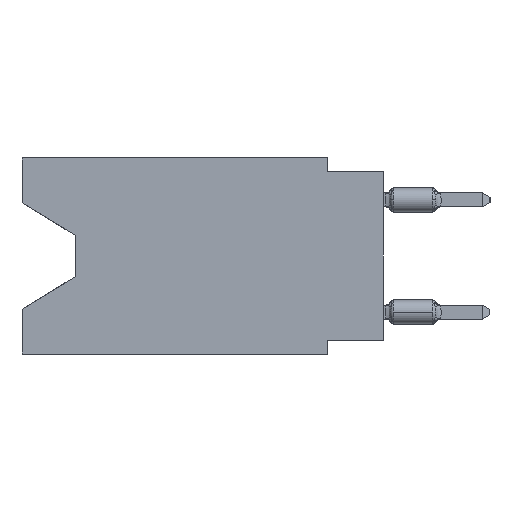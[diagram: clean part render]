
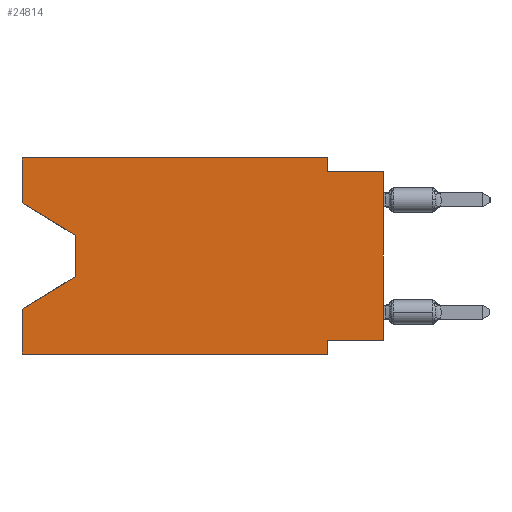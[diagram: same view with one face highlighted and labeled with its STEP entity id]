
A CAD part, left-side view. The second image highlights one B-rep face of the part: STEP entity #24814.
In plain terms, the highlighted planar face has unit normal (-1, 0, 0).
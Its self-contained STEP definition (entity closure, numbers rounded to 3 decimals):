
#382 = ORIENTED_EDGE ( 'NONE', *, *, #13523, .F. ) ;
#453 = ORIENTED_EDGE ( 'NONE', *, *, #15344, .F. ) ;
#481 = VECTOR ( 'NONE', #26315, 1000. ) ;
#1238 = LINE ( 'NONE', #21704, #481 ) ;
#2093 = VECTOR ( 'NONE', #11707, 1000. ) ;
#2851 = ORIENTED_EDGE ( 'NONE', *, *, #11258, .F. ) ;
#3063 = DIRECTION ( 'NONE',  ( 0., 0., -1. ) ) ;
#3077 = EDGE_CURVE ( 'NONE', #9585, #11407, #1238, .T. ) ;
#3196 = ORIENTED_EDGE ( 'NONE', *, *, #18572, .T. ) ;
#3495 = CARTESIAN_POINT ( 'NONE',  ( 0., 2.54, -8.255 ) ) ;
#4495 = DIRECTION ( 'NONE',  ( 0., 0., -1. ) ) ;
#4534 = DIRECTION ( 'NONE',  ( 0., 1., 0. ) ) ;
#4892 = LINE ( 'NONE', #27179, #11054 ) ;
#5324 = DIRECTION ( 'NONE',  ( 0., -1., 0. ) ) ;
#5427 = CARTESIAN_POINT ( 'NONE',  ( 0., 16.383, 0. ) ) ;
#6750 = ORIENTED_EDGE ( 'NONE', *, *, #13107, .F. ) ;
#6770 = CARTESIAN_POINT ( 'NONE',  ( 0., 16.383, 0. ) ) ;
#6858 = FACE_OUTER_BOUND ( 'NONE', #20881, .T. ) ;
#7109 = CARTESIAN_POINT ( 'NONE',  ( 0., 2.54, 0. ) ) ;
#7280 = ORIENTED_EDGE ( 'NONE', *, *, #23712, .F. ) ;
#7559 = CARTESIAN_POINT ( 'NONE',  ( 0., 0., -0.635 ) ) ;
#7583 = VERTEX_POINT ( 'NONE', #18325 ) ;
#8108 = VERTEX_POINT ( 'NONE', #23703 ) ;
#8477 = LINE ( 'NONE', #10928, #9392 ) ;
#8680 = CARTESIAN_POINT ( 'NONE',  ( 0., 16.383, -2.038 ) ) ;
#8782 = DIRECTION ( 'NONE',  ( 0., 0., -1. ) ) ;
#8787 = CARTESIAN_POINT ( 'NONE',  ( 0., 16.383, -8.89 ) ) ;
#8921 = CARTESIAN_POINT ( 'NONE',  ( 0., 13.97, -5.385 ) ) ;
#9138 = VECTOR ( 'NONE', #27898, 1000. ) ;
#9165 = DIRECTION ( 'NONE',  ( 1., 0., 0. ) ) ;
#9356 = ORIENTED_EDGE ( 'NONE', *, *, #18337, .T. ) ;
#9392 = VECTOR ( 'NONE', #8782, 1000. ) ;
#9585 = VERTEX_POINT ( 'NONE', #29245 ) ;
#10157 = DIRECTION ( 'NONE',  ( 0., -1., 0. ) ) ;
#10461 = VERTEX_POINT ( 'NONE', #8787 ) ;
#10928 = CARTESIAN_POINT ( 'NONE',  ( 0., 2.54, -8.89 ) ) ;
#11054 = VECTOR ( 'NONE', #27361, 1000. ) ;
#11258 = EDGE_CURVE ( 'NONE', #10461, #27823, #19086, .T. ) ;
#11407 = VERTEX_POINT ( 'NONE', #7559 ) ;
#11707 = DIRECTION ( 'NONE',  ( 0., 0.855, -0.519 ) ) ;
#11985 = CARTESIAN_POINT ( 'NONE',  ( 0., 16.383, 0. ) ) ;
#12693 = VERTEX_POINT ( 'NONE', #3495 ) ;
#12745 = VECTOR ( 'NONE', #29093, 1000. ) ;
#13041 = VECTOR ( 'NONE', #3063, 1000. ) ;
#13075 = LINE ( 'NONE', #29996, #27755 ) ;
#13107 = EDGE_CURVE ( 'NONE', #21252, #29149, #15743, .T. ) ;
#13523 = EDGE_CURVE ( 'NONE', #23536, #15535, #29579, .T. ) ;
#13585 = LINE ( 'NONE', #8680, #18753 ) ;
#14498 = EDGE_CURVE ( 'NONE', #7583, #29697, #25873, .T. ) ;
#15344 = EDGE_CURVE ( 'NONE', #12693, #8108, #8477, .T. ) ;
#15535 = VERTEX_POINT ( 'NONE', #29745 ) ;
#15743 = LINE ( 'NONE', #5427, #9138 ) ;
#16548 = EDGE_CURVE ( 'NONE', #21252, #7583, #13585, .T. ) ;
#16864 = DIRECTION ( 'NONE',  ( 0., 0., -1. ) ) ;
#16993 = LINE ( 'NONE', #27005, #24701 ) ;
#17126 = ORIENTED_EDGE ( 'NONE', *, *, #25287, .F. ) ;
#17277 = CARTESIAN_POINT ( 'NONE',  ( 0., 16.383, -8.89 ) ) ;
#17345 = AXIS2_PLACEMENT_3D ( 'NONE', #22113, #9165, #16864 ) ;
#18325 = CARTESIAN_POINT ( 'NONE',  ( 0., 13.97, -3.505 ) ) ;
#18337 = EDGE_CURVE ( 'NONE', #10461, #8108, #32209, .T. ) ;
#18572 = EDGE_CURVE ( 'NONE', #29697, #27823, #28940, .T. ) ;
#18753 = VECTOR ( 'NONE', #23597, 1000. ) ;
#19086 = LINE ( 'NONE', #6770, #12745 ) ;
#19570 = ORIENTED_EDGE ( 'NONE', *, *, #29716, .F. ) ;
#19927 = ORIENTED_EDGE ( 'NONE', *, *, #14498, .T. ) ;
#20881 = EDGE_LOOP ( 'NONE', ( #23622, #19927, #3196, #2851, #9356, #453, #17126, #29491, #7280, #382, #19570, #6750 ) ) ;
#21252 = VERTEX_POINT ( 'NONE', #22358 ) ;
#21638 = PLANE ( 'NONE',  #17345 ) ;
#21704 = CARTESIAN_POINT ( 'NONE',  ( 0., 0., 0. ) ) ;
#22113 = CARTESIAN_POINT ( 'NONE',  ( 0., 16.383, 0. ) ) ;
#22358 = CARTESIAN_POINT ( 'NONE',  ( 0., 16.383, -2.038 ) ) ;
#23242 = VECTOR ( 'NONE', #4495, 1000. ) ;
#23536 = VERTEX_POINT ( 'NONE', #26874 ) ;
#23597 = DIRECTION ( 'NONE',  ( 0., -0.855, -0.519 ) ) ;
#23622 = ORIENTED_EDGE ( 'NONE', *, *, #16548, .T. ) ;
#23703 = CARTESIAN_POINT ( 'NONE',  ( 0., 2.54, -8.89 ) ) ;
#23712 = EDGE_CURVE ( 'NONE', #15535, #11407, #4892, .T. ) ;
#24701 = VECTOR ( 'NONE', #4534, 1000. ) ;
#24814 = ADVANCED_FACE ( 'NONE', ( #6858 ), #21638, .F. ) ;
#25287 = EDGE_CURVE ( 'NONE', #9585, #12693, #16993, .T. ) ;
#25535 = CARTESIAN_POINT ( 'NONE',  ( 0., 13.97, -3.505 ) ) ;
#25873 = LINE ( 'NONE', #25535, #13041 ) ;
#25976 = CARTESIAN_POINT ( 'NONE',  ( 0., 16.383, -6.852 ) ) ;
#26315 = DIRECTION ( 'NONE',  ( 0., 0., 1. ) ) ;
#26874 = CARTESIAN_POINT ( 'NONE',  ( 0., 2.54, 0. ) ) ;
#27005 = CARTESIAN_POINT ( 'NONE',  ( 0., 0., -8.255 ) ) ;
#27179 = CARTESIAN_POINT ( 'NONE',  ( 0., 0., -0.635 ) ) ;
#27361 = DIRECTION ( 'NONE',  ( 0., -1., 0. ) ) ;
#27753 = VECTOR ( 'NONE', #5324, 1000. ) ;
#27755 = VECTOR ( 'NONE', #10157, 1000. ) ;
#27823 = VERTEX_POINT ( 'NONE', #25976 ) ;
#27898 = DIRECTION ( 'NONE',  ( 0., 0., 1. ) ) ;
#28034 = CARTESIAN_POINT ( 'NONE',  ( 0., 13.97, -5.385 ) ) ;
#28940 = LINE ( 'NONE', #8921, #2093 ) ;
#29093 = DIRECTION ( 'NONE',  ( 0., 0., 1. ) ) ;
#29149 = VERTEX_POINT ( 'NONE', #11985 ) ;
#29245 = CARTESIAN_POINT ( 'NONE',  ( 0., 0., -8.255 ) ) ;
#29491 = ORIENTED_EDGE ( 'NONE', *, *, #3077, .T. ) ;
#29579 = LINE ( 'NONE', #7109, #23242 ) ;
#29697 = VERTEX_POINT ( 'NONE', #28034 ) ;
#29716 = EDGE_CURVE ( 'NONE', #29149, #23536, #13075, .T. ) ;
#29745 = CARTESIAN_POINT ( 'NONE',  ( 0., 2.54, -0.635 ) ) ;
#29996 = CARTESIAN_POINT ( 'NONE',  ( 0., 16.383, 0. ) ) ;
#32209 = LINE ( 'NONE', #17277, #27753 ) ;
